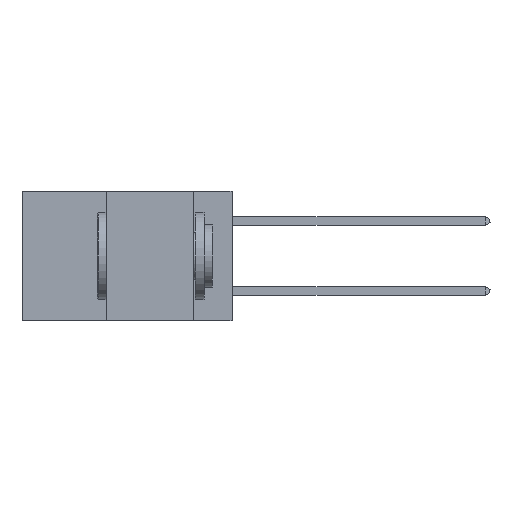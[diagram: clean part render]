
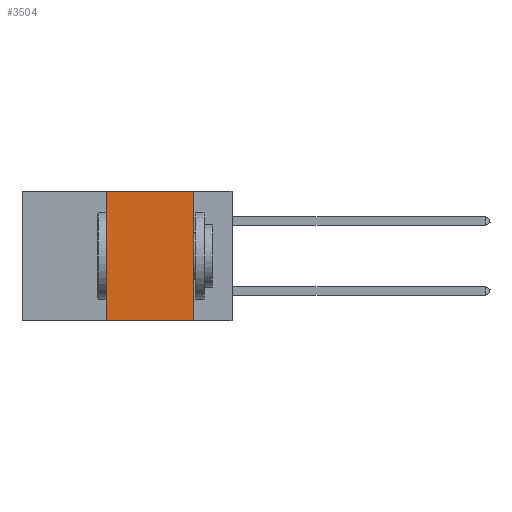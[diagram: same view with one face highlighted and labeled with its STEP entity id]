
A CAD part, left-side view. The second image highlights one B-rep face of the part: STEP entity #3504.
In plain terms, the highlighted planar face has unit normal (-1, 0, 0).
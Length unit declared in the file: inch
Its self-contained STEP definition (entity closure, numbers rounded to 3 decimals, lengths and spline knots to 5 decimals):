
#298 = DIRECTION ( 'NONE',  ( 0., 0., 1. ) ) ;
#901 = CARTESIAN_POINT ( 'NONE',  ( 0., 0.11, -0.37 ) ) ;
#2041 = LINE ( 'NONE', #8349, #23694 ) ;
#3338 = CARTESIAN_POINT ( 'NONE',  ( 0., 0.36, 0. ) ) ;
#3504 = ADVANCED_FACE ( 'NONE', ( #25379 ), #15306, .F. ) ;
#4173 = ORIENTED_EDGE ( 'NONE', *, *, #35909, .F. ) ;
#4354 = VECTOR ( 'NONE', #14322, 39.37008 ) ;
#6598 = EDGE_CURVE ( 'NONE', #12126, #18425, #15418, .T. ) ;
#6939 = EDGE_CURVE ( 'NONE', #12126, #17165, #24993, .T. ) ;
#7609 = DIRECTION ( 'NONE',  ( 0., -1., 0. ) ) ;
#8349 = CARTESIAN_POINT ( 'NONE',  ( 0., 0.11, 0. ) ) ;
#9818 = DIRECTION ( 'NONE',  ( 1., 0., 0. ) ) ;
#10754 = CARTESIAN_POINT ( 'NONE',  ( 0., 0.11, 0. ) ) ;
#11507 = CARTESIAN_POINT ( 'NONE',  ( 0., 0.6, 0. ) ) ;
#12126 = VERTEX_POINT ( 'NONE', #14167 ) ;
#12738 = VECTOR ( 'NONE', #7609, 39.37008 ) ;
#12986 = EDGE_CURVE ( 'NONE', #29008, #17165, #2041, .T. ) ;
#14167 = CARTESIAN_POINT ( 'NONE',  ( 0., 0.36, -0.37 ) ) ;
#14322 = DIRECTION ( 'NONE',  ( 0., -1., 0. ) ) ;
#15306 = PLANE ( 'NONE',  #36203 ) ;
#15418 = LINE ( 'NONE', #28445, #21984 ) ;
#16843 = DIRECTION ( 'NONE',  ( 0., 0., -1. ) ) ;
#17165 = VERTEX_POINT ( 'NONE', #901 ) ;
#18149 = CARTESIAN_POINT ( 'NONE',  ( 0., 0.6, 0. ) ) ;
#18425 = VERTEX_POINT ( 'NONE', #3338 ) ;
#18624 = ORIENTED_EDGE ( 'NONE', *, *, #6939, .T. ) ;
#20682 = EDGE_LOOP ( 'NONE', ( #36124, #4173, #27231, #18624 ) ) ;
#21984 = VECTOR ( 'NONE', #298, 39.37008 ) ;
#23694 = VECTOR ( 'NONE', #16843, 39.37008 ) ;
#24416 = CARTESIAN_POINT ( 'NONE',  ( 0., 0.6, -0.37 ) ) ;
#24993 = LINE ( 'NONE', #24416, #12738 ) ;
#25379 = FACE_OUTER_BOUND ( 'NONE', #20682, .T. ) ;
#26810 = LINE ( 'NONE', #11507, #4354 ) ;
#27231 = ORIENTED_EDGE ( 'NONE', *, *, #6598, .F. ) ;
#28445 = CARTESIAN_POINT ( 'NONE',  ( 0., 0.36, 0. ) ) ;
#29008 = VERTEX_POINT ( 'NONE', #10754 ) ;
#29373 = DIRECTION ( 'NONE',  ( 0., 0., -1. ) ) ;
#35909 = EDGE_CURVE ( 'NONE', #18425, #29008, #26810, .T. ) ;
#36124 = ORIENTED_EDGE ( 'NONE', *, *, #12986, .F. ) ;
#36203 = AXIS2_PLACEMENT_3D ( 'NONE', #18149, #9818, #29373 ) ;
